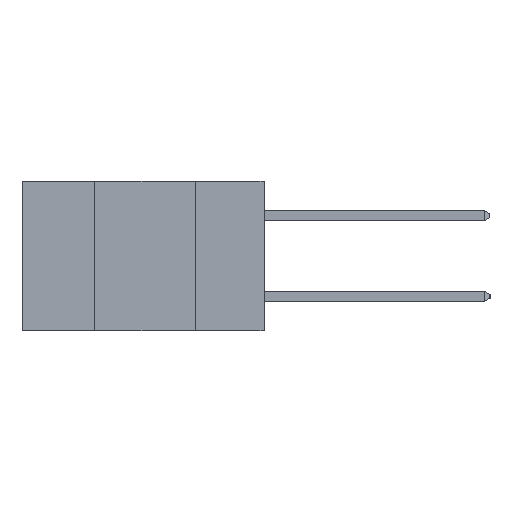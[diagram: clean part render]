
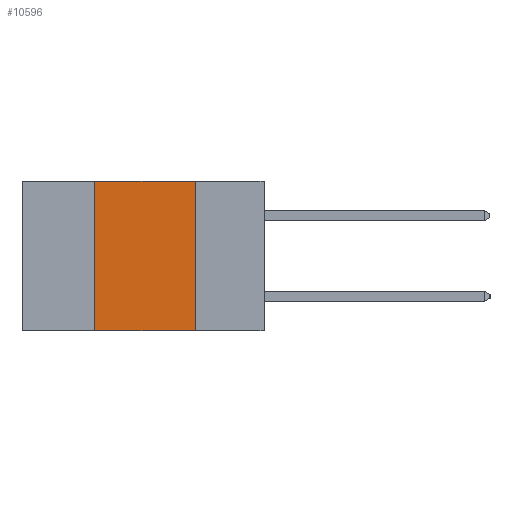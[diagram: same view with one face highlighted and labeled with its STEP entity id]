
A CAD part, left-side view. The second image highlights one B-rep face of the part: STEP entity #10596.
In plain terms, the highlighted planar face has unit normal (-1, 0, 0).
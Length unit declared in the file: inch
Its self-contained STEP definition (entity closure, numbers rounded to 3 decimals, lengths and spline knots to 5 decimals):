
#15 = DIRECTION ( 'NONE',  ( 0., 0., -1. ) ) ;
#97 = VERTEX_POINT ( 'NONE', #10157 ) ;
#212 = EDGE_LOOP ( 'NONE', ( #435, #8341, #12179, #16026 ) ) ;
#435 = ORIENTED_EDGE ( 'NONE', *, *, #5090, .F. ) ;
#960 = CARTESIAN_POINT ( 'NONE',  ( 0., 0.17, -0.37 ) ) ;
#1061 = EDGE_CURVE ( 'NONE', #97, #3403, #13606, .T. ) ;
#1102 = AXIS2_PLACEMENT_3D ( 'NONE', #8039, #18153, #9477 ) ;
#1980 = VERTEX_POINT ( 'NONE', #9321 ) ;
#3076 = EDGE_CURVE ( 'NONE', #97, #3336, #8649, .T. ) ;
#3336 = VERTEX_POINT ( 'NONE', #8219 ) ;
#3403 = VERTEX_POINT ( 'NONE', #6919 ) ;
#4097 = EDGE_CURVE ( 'NONE', #3336, #1980, #15854, .T. ) ;
#5016 = FACE_OUTER_BOUND ( 'NONE', #212, .T. ) ;
#5090 = EDGE_CURVE ( 'NONE', #1980, #3403, #5838, .T. ) ;
#5838 = LINE ( 'NONE', #960, #13100 ) ;
#6919 = CARTESIAN_POINT ( 'NONE',  ( 0., 0.17, -0.37 ) ) ;
#8039 = CARTESIAN_POINT ( 'NONE',  ( 0., 0.6, 0. ) ) ;
#8219 = CARTESIAN_POINT ( 'NONE',  ( 0., 0.42, 0. ) ) ;
#8341 = ORIENTED_EDGE ( 'NONE', *, *, #4097, .F. ) ;
#8649 = LINE ( 'NONE', #12304, #15890 ) ;
#9307 = VECTOR ( 'NONE', #13641, 39.37008 ) ;
#9321 = CARTESIAN_POINT ( 'NONE',  ( 0., 0.17, 0. ) ) ;
#9477 = DIRECTION ( 'NONE',  ( 0., 0., -1. ) ) ;
#10157 = CARTESIAN_POINT ( 'NONE',  ( 0., 0.42, -0.37 ) ) ;
#10596 = ADVANCED_FACE ( 'NONE', ( #5016 ), #10869, .F. ) ;
#10869 = PLANE ( 'NONE',  #1102 ) ;
#12121 = DIRECTION ( 'NONE',  ( 0., 0., 1. ) ) ;
#12179 = ORIENTED_EDGE ( 'NONE', *, *, #3076, .F. ) ;
#12304 = CARTESIAN_POINT ( 'NONE',  ( 0., 0.42, -0.37 ) ) ;
#13100 = VECTOR ( 'NONE', #15, 39.37008 ) ;
#13606 = LINE ( 'NONE', #17945, #9307 ) ;
#13641 = DIRECTION ( 'NONE',  ( 0., -1., 0. ) ) ;
#13652 = DIRECTION ( 'NONE',  ( 0., -1., 0. ) ) ;
#13905 = CARTESIAN_POINT ( 'NONE',  ( 0., 0.6, 0. ) ) ;
#15854 = LINE ( 'NONE', #13905, #18775 ) ;
#15890 = VECTOR ( 'NONE', #12121, 39.37008 ) ;
#16026 = ORIENTED_EDGE ( 'NONE', *, *, #1061, .T. ) ;
#17945 = CARTESIAN_POINT ( 'NONE',  ( 0., 0.6, -0.37 ) ) ;
#18153 = DIRECTION ( 'NONE',  ( 1., 0., 0. ) ) ;
#18775 = VECTOR ( 'NONE', #13652, 39.37008 ) ;
